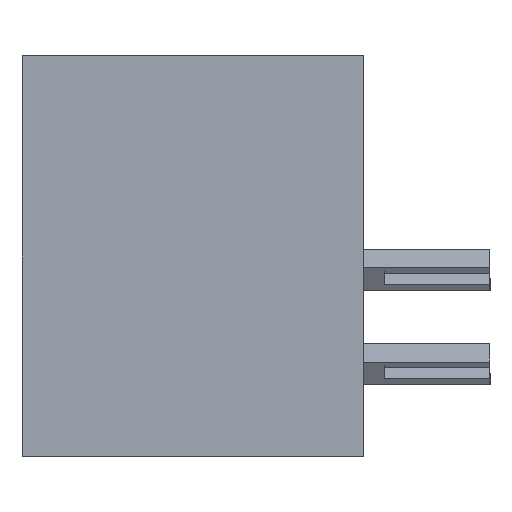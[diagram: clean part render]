
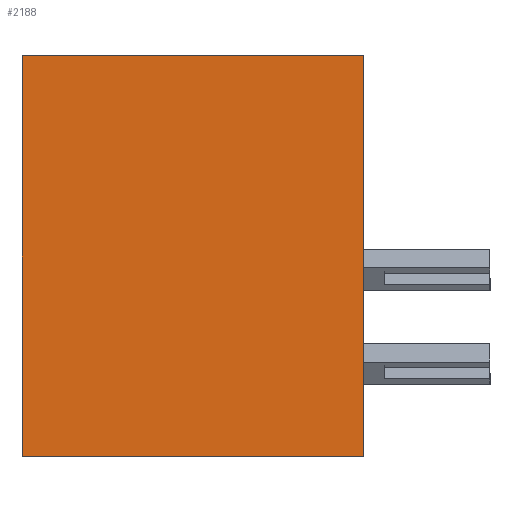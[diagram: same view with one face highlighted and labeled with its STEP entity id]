
A CAD part, left-side view. The second image highlights one B-rep face of the part: STEP entity #2188.
In plain terms, the highlighted planar face has unit normal (-1, 0, 0).
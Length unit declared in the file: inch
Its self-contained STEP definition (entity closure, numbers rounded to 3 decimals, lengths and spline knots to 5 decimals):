
#1079 = LINE ( 'NONE', #13396, #15522 ) ;
#1185 = ORIENTED_EDGE ( 'NONE', *, *, #9549, .T. ) ;
#1807 = EDGE_CURVE ( 'NONE', #10534, #4129, #15130, .T. ) ;
#2188 = ADVANCED_FACE ( 'NONE', ( #5311 ), #16916, .F. ) ;
#2417 = DIRECTION ( 'NONE',  ( 0., -1., 0. ) ) ;
#2479 = CARTESIAN_POINT ( 'NONE',  ( 0., 0.453, 0. ) ) ;
#2924 = DIRECTION ( 'NONE',  ( 0., -1., 0. ) ) ;
#3900 = DIRECTION ( 'NONE',  ( 0., 0., 1. ) ) ;
#4129 = VERTEX_POINT ( 'NONE', #13642 ) ;
#4567 = LINE ( 'NONE', #14483, #8779 ) ;
#4862 = CARTESIAN_POINT ( 'NONE',  ( 0., 0.453, 0. ) ) ;
#5303 = CARTESIAN_POINT ( 'NONE',  ( 0., 0.453, 0. ) ) ;
#5311 = FACE_OUTER_BOUND ( 'NONE', #17969, .T. ) ;
#5510 = LINE ( 'NONE', #5303, #16705 ) ;
#5881 = VERTEX_POINT ( 'NONE', #9228 ) ;
#7761 = DIRECTION ( 'NONE',  ( 0., 0., -1. ) ) ;
#8779 = VECTOR ( 'NONE', #15714, 39.37008 ) ;
#8882 = ORIENTED_EDGE ( 'NONE', *, *, #9106, .T. ) ;
#9106 = EDGE_CURVE ( 'NONE', #5881, #10011, #1079, .T. ) ;
#9228 = CARTESIAN_POINT ( 'NONE',  ( 0., 0.453, -0.531 ) ) ;
#9549 = EDGE_CURVE ( 'NONE', #10011, #4129, #4567, .T. ) ;
#10011 = VERTEX_POINT ( 'NONE', #12207 ) ;
#10241 = VECTOR ( 'NONE', #2417, 39.37008 ) ;
#10534 = VERTEX_POINT ( 'NONE', #13836 ) ;
#12201 = ORIENTED_EDGE ( 'NONE', *, *, #1807, .F. ) ;
#12207 = CARTESIAN_POINT ( 'NONE',  ( 0., 0., -0.531 ) ) ;
#13396 = CARTESIAN_POINT ( 'NONE',  ( 0., 0.453, -0.531 ) ) ;
#13642 = CARTESIAN_POINT ( 'NONE',  ( 0., 0., 0. ) ) ;
#13836 = CARTESIAN_POINT ( 'NONE',  ( 0., 0.453, 0. ) ) ;
#14483 = CARTESIAN_POINT ( 'NONE',  ( 0., 0., 0. ) ) ;
#15130 = LINE ( 'NONE', #2479, #10241 ) ;
#15286 = DIRECTION ( 'NONE',  ( 1., 0., 0. ) ) ;
#15522 = VECTOR ( 'NONE', #2924, 39.37008 ) ;
#15714 = DIRECTION ( 'NONE',  ( 0., 0., 1. ) ) ;
#16580 = ORIENTED_EDGE ( 'NONE', *, *, #17128, .F. ) ;
#16705 = VECTOR ( 'NONE', #3900, 39.37008 ) ;
#16916 = PLANE ( 'NONE',  #18459 ) ;
#17128 = EDGE_CURVE ( 'NONE', #5881, #10534, #5510, .T. ) ;
#17969 = EDGE_LOOP ( 'NONE', ( #1185, #12201, #16580, #8882 ) ) ;
#18459 = AXIS2_PLACEMENT_3D ( 'NONE', #4862, #15286, #7761 ) ;
